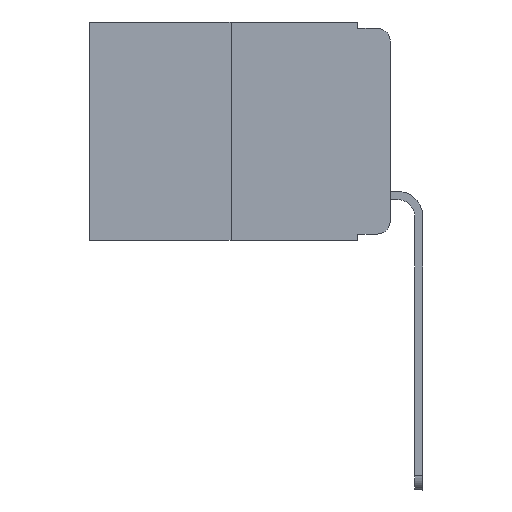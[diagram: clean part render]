
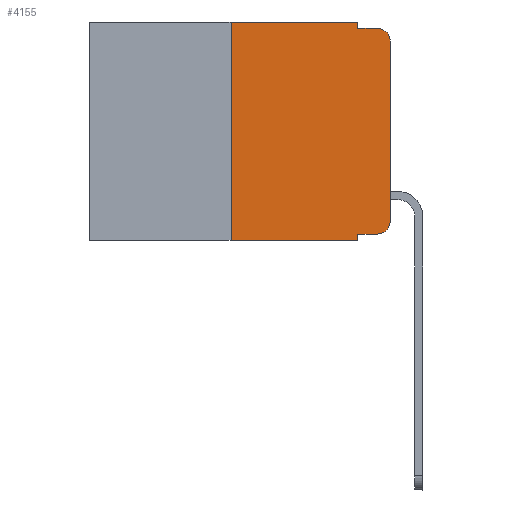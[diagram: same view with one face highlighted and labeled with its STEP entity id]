
A CAD part, left-side view. The second image highlights one B-rep face of the part: STEP entity #4155.
In plain terms, the highlighted planar face has unit normal (-1, 0, 0).
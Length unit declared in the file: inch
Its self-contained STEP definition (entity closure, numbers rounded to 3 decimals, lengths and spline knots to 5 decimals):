
#155 = EDGE_CURVE ( 'NONE', #11025, #5928, #5597, .T. ) ;
#236 = AXIS2_PLACEMENT_3D ( 'NONE', #9172, #6172, #5023 ) ;
#1149 = AXIS2_PLACEMENT_3D ( 'NONE', #12526, #16247, #16337 ) ;
#1196 = DIRECTION ( 'NONE',  ( 0., -1., 0. ) ) ;
#1321 = ORIENTED_EDGE ( 'NONE', *, *, #8570, .T. ) ;
#1471 = ORIENTED_EDGE ( 'NONE', *, *, #13911, .F. ) ;
#1641 = CARTESIAN_POINT ( 'NONE',  ( 0., 0.051, -0.333 ) ) ;
#1774 = DIRECTION ( 'NONE',  ( 0., -1., 0. ) ) ;
#2103 = VECTOR ( 'NONE', #13097, 39.37008 ) ;
#2433 = VERTEX_POINT ( 'NONE', #6919 ) ;
#2932 = EDGE_CURVE ( 'NONE', #9106, #14867, #16264, .T. ) ;
#3484 = VERTEX_POINT ( 'NONE', #16828 ) ;
#3668 = CARTESIAN_POINT ( 'NONE',  ( 0., 0.051, -0.343 ) ) ;
#3785 = CARTESIAN_POINT ( 'NONE',  ( 0., 0.25, 0. ) ) ;
#4087 = PLANE ( 'NONE',  #16336 ) ;
#4155 = ADVANCED_FACE ( 'NONE', ( #6665 ), #4087, .F. ) ;
#4692 = EDGE_CURVE ( 'NONE', #2433, #5928, #9717, .T. ) ;
#4956 = ORIENTED_EDGE ( 'NONE', *, *, #6336, .T. ) ;
#5023 = DIRECTION ( 'NONE',  ( 0., 0., -1. ) ) ;
#5079 = LINE ( 'NONE', #6758, #15098 ) ;
#5102 = VECTOR ( 'NONE', #15165, 39.37008 ) ;
#5597 = CIRCLE ( 'NONE', #236, 0.02 ) ;
#5691 = LINE ( 'NONE', #7109, #16829 ) ;
#5928 = VERTEX_POINT ( 'NONE', #15124 ) ;
#6150 = ORIENTED_EDGE ( 'NONE', *, *, #13889, .F. ) ;
#6172 = DIRECTION ( 'NONE',  ( -1., 0., 0. ) ) ;
#6336 = EDGE_CURVE ( 'NONE', #3484, #16235, #10145, .T. ) ;
#6409 = CARTESIAN_POINT ( 'NONE',  ( 0., 0.051, 0. ) ) ;
#6665 = FACE_OUTER_BOUND ( 'NONE', #7358, .T. ) ;
#6683 = CARTESIAN_POINT ( 'NONE',  ( 0., 0., -0.313 ) ) ;
#6758 = CARTESIAN_POINT ( 'NONE',  ( 0., 0.473, 0. ) ) ;
#6919 = CARTESIAN_POINT ( 'NONE',  ( 0., 0.051, -0.01 ) ) ;
#7025 = DIRECTION ( 'NONE',  ( 0., -1., 0. ) ) ;
#7109 = CARTESIAN_POINT ( 'NONE',  ( 0., 0.25, 0. ) ) ;
#7358 = EDGE_LOOP ( 'NONE', ( #1321, #11061, #12350, #1471, #6150, #11761, #14383, #11941, #12950, #4956 ) ) ;
#8048 = DIRECTION ( 'NONE',  ( 0., 0., -1. ) ) ;
#8262 = DIRECTION ( 'NONE',  ( 0., 0., 1. ) ) ;
#8334 = VECTOR ( 'NONE', #17288, 39.37008 ) ;
#8570 = EDGE_CURVE ( 'NONE', #16235, #11025, #16487, .T. ) ;
#9031 = CARTESIAN_POINT ( 'NONE',  ( 0., 0.473, -0.343 ) ) ;
#9106 = VERTEX_POINT ( 'NONE', #12803 ) ;
#9172 = CARTESIAN_POINT ( 'NONE',  ( 0., 0.02, -0.03 ) ) ;
#9221 = DIRECTION ( 'NONE',  ( 1., 0., 0. ) ) ;
#9717 = LINE ( 'NONE', #15030, #17266 ) ;
#9766 = CARTESIAN_POINT ( 'NONE',  ( 0., 0., 0. ) ) ;
#10145 = CIRCLE ( 'NONE', #1149, 0.02 ) ;
#10422 = VERTEX_POINT ( 'NONE', #15644 ) ;
#10902 = VECTOR ( 'NONE', #7025, 39.37008 ) ;
#11025 = VERTEX_POINT ( 'NONE', #13578 ) ;
#11061 = ORIENTED_EDGE ( 'NONE', *, *, #155, .T. ) ;
#11118 = VECTOR ( 'NONE', #8048, 39.37008 ) ;
#11742 = EDGE_CURVE ( 'NONE', #17416, #14867, #11783, .T. ) ;
#11761 = ORIENTED_EDGE ( 'NONE', *, *, #15157, .F. ) ;
#11783 = LINE ( 'NONE', #9031, #2103 ) ;
#11795 = DIRECTION ( 'NONE',  ( 0., 0., -1. ) ) ;
#11860 = CARTESIAN_POINT ( 'NONE',  ( 0., 0.051, 0. ) ) ;
#11941 = ORIENTED_EDGE ( 'NONE', *, *, #2932, .F. ) ;
#12350 = ORIENTED_EDGE ( 'NONE', *, *, #4692, .F. ) ;
#12526 = CARTESIAN_POINT ( 'NONE',  ( 0., 0.02, -0.313 ) ) ;
#12803 = CARTESIAN_POINT ( 'NONE',  ( 0., 0.051, -0.333 ) ) ;
#12950 = ORIENTED_EDGE ( 'NONE', *, *, #15253, .T. ) ;
#13046 = CARTESIAN_POINT ( 'NONE',  ( 0., 0.25, -0.343 ) ) ;
#13097 = DIRECTION ( 'NONE',  ( 0., -1., 0. ) ) ;
#13578 = CARTESIAN_POINT ( 'NONE',  ( 0., 0., -0.03 ) ) ;
#13738 = LINE ( 'NONE', #1641, #10902 ) ;
#13889 = EDGE_CURVE ( 'NONE', #17036, #10422, #5079, .T. ) ;
#13911 = EDGE_CURVE ( 'NONE', #10422, #2433, #14624, .T. ) ;
#14383 = ORIENTED_EDGE ( 'NONE', *, *, #11742, .T. ) ;
#14624 = LINE ( 'NONE', #6409, #8334 ) ;
#14867 = VERTEX_POINT ( 'NONE', #3668 ) ;
#15030 = CARTESIAN_POINT ( 'NONE',  ( 0., 0.051, -0.01 ) ) ;
#15098 = VECTOR ( 'NONE', #1196, 39.37008 ) ;
#15124 = CARTESIAN_POINT ( 'NONE',  ( 0., 0.02, -0.01 ) ) ;
#15157 = EDGE_CURVE ( 'NONE', #17416, #17036, #5691, .T. ) ;
#15165 = DIRECTION ( 'NONE',  ( 0., 0., 1. ) ) ;
#15253 = EDGE_CURVE ( 'NONE', #9106, #3484, #13738, .T. ) ;
#15644 = CARTESIAN_POINT ( 'NONE',  ( 0., 0.051, 0. ) ) ;
#15848 = CARTESIAN_POINT ( 'NONE',  ( 0., 0.473, 0. ) ) ;
#16235 = VERTEX_POINT ( 'NONE', #6683 ) ;
#16247 = DIRECTION ( 'NONE',  ( -1., 0., 0. ) ) ;
#16264 = LINE ( 'NONE', #11860, #11118 ) ;
#16336 = AXIS2_PLACEMENT_3D ( 'NONE', #15848, #9221, #11795 ) ;
#16337 = DIRECTION ( 'NONE',  ( 0., 0., -1. ) ) ;
#16487 = LINE ( 'NONE', #9766, #5102 ) ;
#16828 = CARTESIAN_POINT ( 'NONE',  ( 0., 0.02, -0.333 ) ) ;
#16829 = VECTOR ( 'NONE', #8262, 39.37008 ) ;
#17036 = VERTEX_POINT ( 'NONE', #3785 ) ;
#17266 = VECTOR ( 'NONE', #1774, 39.37008 ) ;
#17288 = DIRECTION ( 'NONE',  ( 0., 0., -1. ) ) ;
#17416 = VERTEX_POINT ( 'NONE', #13046 ) ;
